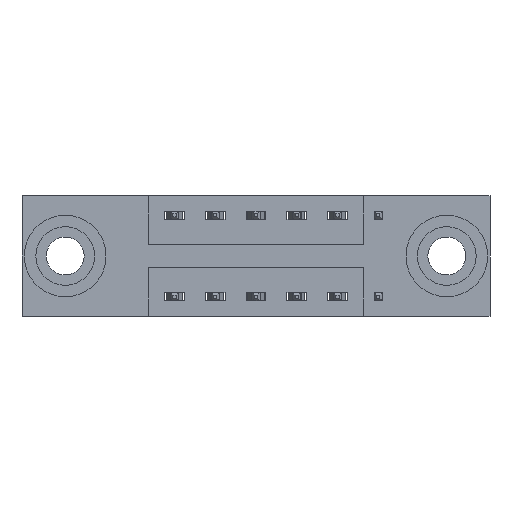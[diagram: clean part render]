
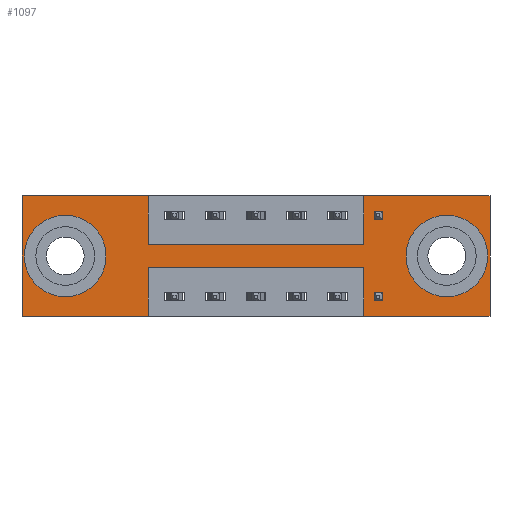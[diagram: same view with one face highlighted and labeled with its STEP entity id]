
A CAD part, front view. The second image highlights one B-rep face of the part: STEP entity #1097.
In plain terms, the highlighted planar face has unit normal (0, -1, 0).
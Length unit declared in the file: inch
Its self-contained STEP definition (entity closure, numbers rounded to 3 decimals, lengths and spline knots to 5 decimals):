
#9 = CARTESIAN_POINT ( 'NONE',  ( 1.3025, 0., -0.185 ) ) ;
#77 = CARTESIAN_POINT ( 'NONE',  ( 0.3875, 0., -0.37 ) ) ;
#133 = CIRCLE ( 'NONE', #6365, 0.078 ) ;
#148 = VERTEX_POINT ( 'NONE', #8640 ) ;
#249 = ORIENTED_EDGE ( 'NONE', *, *, #6001, .T. ) ;
#302 = CARTESIAN_POINT ( 'NONE',  ( 1.0475, 0., 0. ) ) ;
#356 = VERTEX_POINT ( 'NONE', #7935 ) ;
#382 = CARTESIAN_POINT ( 'NONE',  ( 0., 0., 0. ) ) ;
#453 = CARTESIAN_POINT ( 'NONE',  ( 0.1325, 0., -0.185 ) ) ;
#571 = DIRECTION ( 'NONE',  ( 0., 0., -1. ) ) ;
#686 = CARTESIAN_POINT ( 'NONE',  ( 0., 0., -0.37 ) ) ;
#798 = VERTEX_POINT ( 'NONE', #3152 ) ;
#830 = VECTOR ( 'NONE', #1493, 39.37008 ) ;
#832 = AXIS2_PLACEMENT_3D ( 'NONE', #4319, #7186, #571 ) ;
#833 = DIRECTION ( 'NONE',  ( 0., 0., 1. ) ) ;
#900 = CARTESIAN_POINT ( 'NONE',  ( 0., 0., 0. ) ) ;
#956 = ORIENTED_EDGE ( 'NONE', *, *, #1810, .F. ) ;
#1031 = ORIENTED_EDGE ( 'NONE', *, *, #8478, .F. ) ;
#1097 = ADVANCED_FACE ( 'NONE', ( #7092, #5044, #1391 ), #7938, .T. ) ;
#1345 = CIRCLE ( 'NONE', #2532, 0.078 ) ;
#1391 = FACE_OUTER_BOUND ( 'NONE', #5349, .T. ) ;
#1493 = DIRECTION ( 'NONE',  ( 0., 0., 1. ) ) ;
#1532 = EDGE_CURVE ( 'NONE', #4565, #798, #5584, .T. ) ;
#1639 = VECTOR ( 'NONE', #7421, 39.37008 ) ;
#1755 = VECTOR ( 'NONE', #6729, 39.37008 ) ;
#1810 = EDGE_CURVE ( 'NONE', #6199, #4908, #8097, .T. ) ;
#1852 = VERTEX_POINT ( 'NONE', #5779 ) ;
#1862 = CARTESIAN_POINT ( 'NONE',  ( 1.3025, 0., -0.263 ) ) ;
#1874 = EDGE_CURVE ( 'NONE', #356, #6199, #6598, .T. ) ;
#1914 = DIRECTION ( 'NONE',  ( 1., 0., 0. ) ) ;
#1953 = DIRECTION ( 'NONE',  ( 0., 1., 0. ) ) ;
#2003 = CARTESIAN_POINT ( 'NONE',  ( 0., 0., 0. ) ) ;
#2076 = DIRECTION ( 'NONE',  ( -1., 0., 0. ) ) ;
#2120 = LINE ( 'NONE', #77, #6546 ) ;
#2368 = LINE ( 'NONE', #3214, #1755 ) ;
#2464 = ORIENTED_EDGE ( 'NONE', *, *, #9111, .T. ) ;
#2532 = AXIS2_PLACEMENT_3D ( 'NONE', #7471, #4292, #3403 ) ;
#2550 = DIRECTION ( 'NONE',  ( 0., 0., 1. ) ) ;
#2782 = CARTESIAN_POINT ( 'NONE',  ( 0., 0., -0.37 ) ) ;
#2820 = VERTEX_POINT ( 'NONE', #8524 ) ;
#2855 = CARTESIAN_POINT ( 'NONE',  ( 1.0475, 0., 0. ) ) ;
#2904 = DIRECTION ( 'NONE',  ( 0., 1., 0. ) ) ;
#3024 = CIRCLE ( 'NONE', #4237, 0.078 ) ;
#3070 = CARTESIAN_POINT ( 'NONE',  ( 1.0475, 0., -0.15 ) ) ;
#3152 = CARTESIAN_POINT ( 'NONE',  ( 1.435, 0., -0.37 ) ) ;
#3214 = CARTESIAN_POINT ( 'NONE',  ( 0.3875, 0., -0.22 ) ) ;
#3259 = EDGE_CURVE ( 'NONE', #7293, #1852, #2368, .T. ) ;
#3342 = LINE ( 'NONE', #2003, #8312 ) ;
#3361 = CARTESIAN_POINT ( 'NONE',  ( 1.435, 0., 0. ) ) ;
#3399 = VECTOR ( 'NONE', #7161, 39.37008 ) ;
#3403 = DIRECTION ( 'NONE',  ( 0., 0., -1. ) ) ;
#3506 = LINE ( 'NONE', #2782, #5928 ) ;
#3616 = DIRECTION ( 'NONE',  ( 0., 0., 1. ) ) ;
#3692 = LINE ( 'NONE', #900, #1639 ) ;
#3897 = EDGE_CURVE ( 'NONE', #6512, #7293, #5733, .T. ) ;
#3942 = ORIENTED_EDGE ( 'NONE', *, *, #1874, .F. ) ;
#4013 = VERTEX_POINT ( 'NONE', #7629 ) ;
#4030 = ORIENTED_EDGE ( 'NONE', *, *, #7945, .F. ) ;
#4058 = VECTOR ( 'NONE', #8007, 39.37008 ) ;
#4237 = AXIS2_PLACEMENT_3D ( 'NONE', #9, #2904, #5828 ) ;
#4290 = LINE ( 'NONE', #686, #4058 ) ;
#4292 = DIRECTION ( 'NONE',  ( 0., 1., 0. ) ) ;
#4319 = CARTESIAN_POINT ( 'NONE',  ( 0., 0., -0.37 ) ) ;
#4409 = AXIS2_PLACEMENT_3D ( 'NONE', #453, #7017, #7671 ) ;
#4565 = VERTEX_POINT ( 'NONE', #3361 ) ;
#4830 = ORIENTED_EDGE ( 'NONE', *, *, #1532, .F. ) ;
#4895 = VERTEX_POINT ( 'NONE', #8861 ) ;
#4908 = VERTEX_POINT ( 'NONE', #302 ) ;
#4920 = CARTESIAN_POINT ( 'NONE',  ( 0.3875, 0., 0. ) ) ;
#5044 = FACE_BOUND ( 'NONE', #5809, .T. ) ;
#5251 = VECTOR ( 'NONE', #7527, 39.37008 ) ;
#5347 = VERTEX_POINT ( 'NONE', #6368 ) ;
#5349 = EDGE_LOOP ( 'NONE', ( #5822, #8341, #8119, #1031, #4830, #8602, #956, #3942, #4030, #8191, #5390, #8547 ) ) ;
#5390 = ORIENTED_EDGE ( 'NONE', *, *, #6267, .F. ) ;
#5512 = LINE ( 'NONE', #382, #7552 ) ;
#5584 = LINE ( 'NONE', #9209, #3399 ) ;
#5605 = CARTESIAN_POINT ( 'NONE',  ( 0.3875, 0., -0.15 ) ) ;
#5658 = EDGE_CURVE ( 'NONE', #9240, #4895, #3342, .T. ) ;
#5733 = LINE ( 'NONE', #6704, #6853 ) ;
#5779 = CARTESIAN_POINT ( 'NONE',  ( 0.3875, 0., -0.22 ) ) ;
#5809 = EDGE_LOOP ( 'NONE', ( #2464, #8988 ) ) ;
#5822 = ORIENTED_EDGE ( 'NONE', *, *, #8957, .F. ) ;
#5827 = LINE ( 'NONE', #4920, #8023 ) ;
#5828 = DIRECTION ( 'NONE',  ( 0., 0., -1. ) ) ;
#5928 = VECTOR ( 'NONE', #2076, 39.37008 ) ;
#6001 = EDGE_CURVE ( 'NONE', #9173, #4013, #1345, .T. ) ;
#6199 = VERTEX_POINT ( 'NONE', #3070 ) ;
#6267 = EDGE_CURVE ( 'NONE', #148, #9240, #5512, .T. ) ;
#6365 = AXIS2_PLACEMENT_3D ( 'NONE', #7061, #1953, #3616 ) ;
#6368 = CARTESIAN_POINT ( 'NONE',  ( 0.1325, 0., -0.107 ) ) ;
#6488 = EDGE_CURVE ( 'NONE', #4908, #4565, #3692, .T. ) ;
#6512 = VERTEX_POINT ( 'NONE', #6630 ) ;
#6546 = VECTOR ( 'NONE', #7222, 39.37008 ) ;
#6598 = LINE ( 'NONE', #5605, #5251 ) ;
#6630 = CARTESIAN_POINT ( 'NONE',  ( 1.0475, 0., -0.37 ) ) ;
#6704 = CARTESIAN_POINT ( 'NONE',  ( 1.0475, 0., -0.37 ) ) ;
#6729 = DIRECTION ( 'NONE',  ( -1., 0., 0. ) ) ;
#6853 = VECTOR ( 'NONE', #833, 39.37008 ) ;
#7017 = DIRECTION ( 'NONE',  ( 0., 1., 0. ) ) ;
#7061 = CARTESIAN_POINT ( 'NONE',  ( 0.1325, 0., -0.185 ) ) ;
#7092 = FACE_BOUND ( 'NONE', #7178, .T. ) ;
#7150 = CARTESIAN_POINT ( 'NONE',  ( 0., 0., 0. ) ) ;
#7161 = DIRECTION ( 'NONE',  ( 0., 0., -1. ) ) ;
#7178 = EDGE_LOOP ( 'NONE', ( #7530, #249 ) ) ;
#7186 = DIRECTION ( 'NONE',  ( 0., -1., 0. ) ) ;
#7222 = DIRECTION ( 'NONE',  ( 0., 0., -1. ) ) ;
#7293 = VERTEX_POINT ( 'NONE', #7457 ) ;
#7421 = DIRECTION ( 'NONE',  ( 1., 0., 0. ) ) ;
#7457 = CARTESIAN_POINT ( 'NONE',  ( 1.0475, 0., -0.22 ) ) ;
#7471 = CARTESIAN_POINT ( 'NONE',  ( 1.3025, 0., -0.185 ) ) ;
#7527 = DIRECTION ( 'NONE',  ( 1., 0., 0. ) ) ;
#7530 = ORIENTED_EDGE ( 'NONE', *, *, #9375, .T. ) ;
#7552 = VECTOR ( 'NONE', #2550, 39.37008 ) ;
#7571 = EDGE_CURVE ( 'NONE', #7931, #148, #4290, .T. ) ;
#7629 = CARTESIAN_POINT ( 'NONE',  ( 1.3025, 0., -0.107 ) ) ;
#7671 = DIRECTION ( 'NONE',  ( 0., 0., 1. ) ) ;
#7760 = CARTESIAN_POINT ( 'NONE',  ( 0.3875, 0., -0.37 ) ) ;
#7931 = VERTEX_POINT ( 'NONE', #7760 ) ;
#7935 = CARTESIAN_POINT ( 'NONE',  ( 0.3875, 0., -0.15 ) ) ;
#7938 = PLANE ( 'NONE',  #832 ) ;
#7945 = EDGE_CURVE ( 'NONE', #4895, #356, #5827, .T. ) ;
#7946 = DIRECTION ( 'NONE',  ( 0., 0., -1. ) ) ;
#7979 = EDGE_CURVE ( 'NONE', #2820, #5347, #133, .T. ) ;
#8007 = DIRECTION ( 'NONE',  ( -1., 0., 0. ) ) ;
#8023 = VECTOR ( 'NONE', #7946, 39.37008 ) ;
#8097 = LINE ( 'NONE', #2855, #830 ) ;
#8119 = ORIENTED_EDGE ( 'NONE', *, *, #3897, .F. ) ;
#8191 = ORIENTED_EDGE ( 'NONE', *, *, #5658, .F. ) ;
#8312 = VECTOR ( 'NONE', #1914, 39.37008 ) ;
#8341 = ORIENTED_EDGE ( 'NONE', *, *, #3259, .F. ) ;
#8478 = EDGE_CURVE ( 'NONE', #798, #6512, #3506, .T. ) ;
#8524 = CARTESIAN_POINT ( 'NONE',  ( 0.1325, 0., -0.263 ) ) ;
#8547 = ORIENTED_EDGE ( 'NONE', *, *, #7571, .F. ) ;
#8602 = ORIENTED_EDGE ( 'NONE', *, *, #6488, .F. ) ;
#8640 = CARTESIAN_POINT ( 'NONE',  ( 0., 0., -0.37 ) ) ;
#8861 = CARTESIAN_POINT ( 'NONE',  ( 0.3875, 0., 0. ) ) ;
#8957 = EDGE_CURVE ( 'NONE', #1852, #7931, #2120, .T. ) ;
#8988 = ORIENTED_EDGE ( 'NONE', *, *, #7979, .T. ) ;
#9111 = EDGE_CURVE ( 'NONE', #5347, #2820, #9268, .T. ) ;
#9173 = VERTEX_POINT ( 'NONE', #1862 ) ;
#9209 = CARTESIAN_POINT ( 'NONE',  ( 1.435, 0., 0. ) ) ;
#9240 = VERTEX_POINT ( 'NONE', #7150 ) ;
#9268 = CIRCLE ( 'NONE', #4409, 0.078 ) ;
#9375 = EDGE_CURVE ( 'NONE', #4013, #9173, #3024, .T. ) ;
